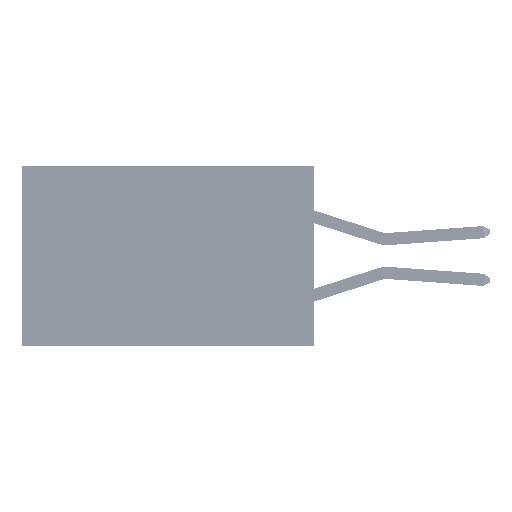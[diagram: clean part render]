
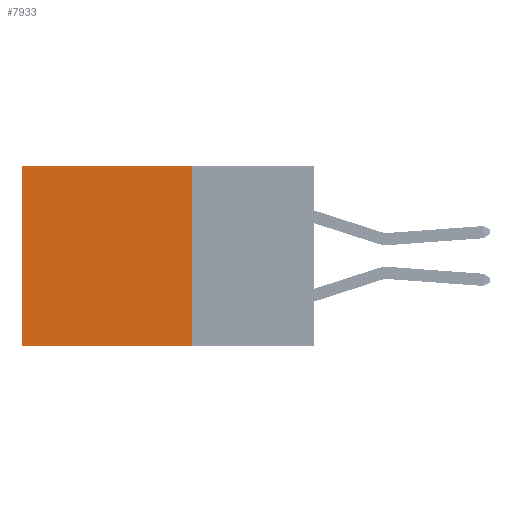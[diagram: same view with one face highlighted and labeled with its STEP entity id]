
A CAD part, left-side view. The second image highlights one B-rep face of the part: STEP entity #7933.
In plain terms, the highlighted planar face has unit normal (-1, 0, 0).
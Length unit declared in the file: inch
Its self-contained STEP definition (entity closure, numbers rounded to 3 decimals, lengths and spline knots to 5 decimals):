
#659 = CARTESIAN_POINT ( 'NONE',  ( 0.2875, 0.25, 0. ) ) ;
#3052 = LINE ( 'NONE', #659, #5295 ) ;
#3549 = CARTESIAN_POINT ( 'NONE',  ( 0.2875, 0.6, 0. ) ) ;
#3617 = LINE ( 'NONE', #3549, #35253 ) ;
#4511 = CARTESIAN_POINT ( 'NONE',  ( 0.2875, 0.25, 0. ) ) ;
#4929 = CARTESIAN_POINT ( 'NONE',  ( 0.2875, 0.25, -0.37 ) ) ;
#5295 = VECTOR ( 'NONE', #32968, 39.37008 ) ;
#5979 = LINE ( 'NONE', #41106, #14460 ) ;
#7171 = DIRECTION ( 'NONE',  ( 0., 0., -1. ) ) ;
#7933 = ADVANCED_FACE ( 'NONE', ( #18589 ), #44247, .F. ) ;
#8158 = CARTESIAN_POINT ( 'NONE',  ( 0.2875, 0.25, -0.37 ) ) ;
#8192 = CARTESIAN_POINT ( 'NONE',  ( 0.2875, 0.6, 0. ) ) ;
#9195 = VERTEX_POINT ( 'NONE', #8192 ) ;
#12464 = AXIS2_PLACEMENT_3D ( 'NONE', #26265, #33654, #15687 ) ;
#13832 = VERTEX_POINT ( 'NONE', #25755 ) ;
#14387 = ORIENTED_EDGE ( 'NONE', *, *, #46635, .F. ) ;
#14460 = VECTOR ( 'NONE', #37023, 39.37008 ) ;
#15369 = EDGE_CURVE ( 'NONE', #22265, #9195, #5979, .T. ) ;
#15687 = DIRECTION ( 'NONE',  ( 0., 0., -1. ) ) ;
#16019 = VERTEX_POINT ( 'NONE', #4929 ) ;
#18589 = FACE_OUTER_BOUND ( 'NONE', #25350, .T. ) ;
#21128 = LINE ( 'NONE', #8158, #42048 ) ;
#22265 = VERTEX_POINT ( 'NONE', #4511 ) ;
#25350 = EDGE_LOOP ( 'NONE', ( #29143, #29244, #14387, #36794 ) ) ;
#25755 = CARTESIAN_POINT ( 'NONE',  ( 0.2875, 0.6, -0.37 ) ) ;
#26265 = CARTESIAN_POINT ( 'NONE',  ( 0.2875, 0.25, 0. ) ) ;
#29143 = ORIENTED_EDGE ( 'NONE', *, *, #34386, .T. ) ;
#29244 = ORIENTED_EDGE ( 'NONE', *, *, #33923, .F. ) ;
#32968 = DIRECTION ( 'NONE',  ( 0., 0., -1. ) ) ;
#33654 = DIRECTION ( 'NONE',  ( 1., 0., 0. ) ) ;
#33680 = DIRECTION ( 'NONE',  ( 0., 1., 0. ) ) ;
#33923 = EDGE_CURVE ( 'NONE', #16019, #13832, #21128, .T. ) ;
#34386 = EDGE_CURVE ( 'NONE', #9195, #13832, #3617, .T. ) ;
#35253 = VECTOR ( 'NONE', #7171, 39.37008 ) ;
#36794 = ORIENTED_EDGE ( 'NONE', *, *, #15369, .T. ) ;
#37023 = DIRECTION ( 'NONE',  ( 0., 1., 0. ) ) ;
#41106 = CARTESIAN_POINT ( 'NONE',  ( 0.2875, 0.25, 0. ) ) ;
#42048 = VECTOR ( 'NONE', #33680, 39.37008 ) ;
#44247 = PLANE ( 'NONE',  #12464 ) ;
#46635 = EDGE_CURVE ( 'NONE', #22265, #16019, #3052, .T. ) ;
